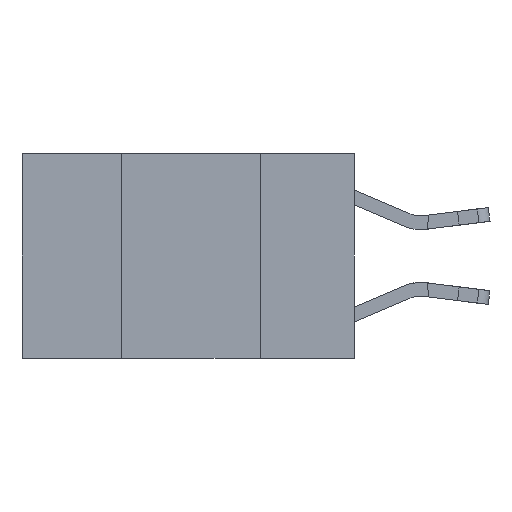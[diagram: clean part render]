
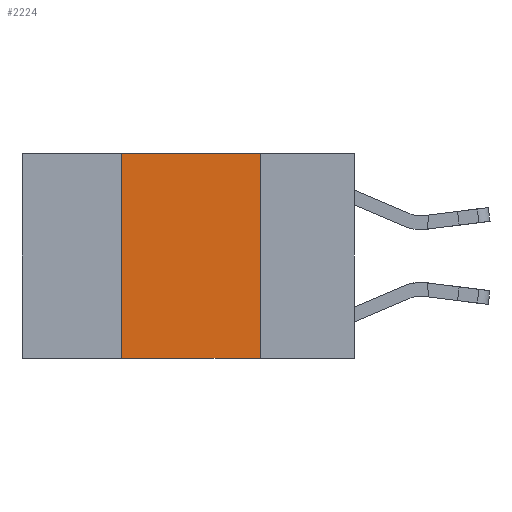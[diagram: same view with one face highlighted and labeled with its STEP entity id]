
A CAD part, left-side view. The second image highlights one B-rep face of the part: STEP entity #2224.
In plain terms, the highlighted planar face has unit normal (-1, 0, 0).
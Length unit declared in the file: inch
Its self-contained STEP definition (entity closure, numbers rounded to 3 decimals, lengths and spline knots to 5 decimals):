
#190 = CARTESIAN_POINT ( 'NONE',  ( 0., 0.17, -0.37 ) ) ;
#291 = VECTOR ( 'NONE', #15380, 39.37008 ) ;
#1201 = AXIS2_PLACEMENT_3D ( 'NONE', #17221, #19103, #23726 ) ;
#1230 = VERTEX_POINT ( 'NONE', #17264 ) ;
#2224 = ADVANCED_FACE ( 'NONE', ( #10831 ), #8373, .F. ) ;
#3230 = EDGE_CURVE ( 'NONE', #23734, #20694, #17258, .T. ) ;
#4207 = ORIENTED_EDGE ( 'NONE', *, *, #10523, .T. ) ;
#4534 = ORIENTED_EDGE ( 'NONE', *, *, #9745, .F. ) ;
#5258 = CARTESIAN_POINT ( 'NONE',  ( 0., 0.6, -0.37 ) ) ;
#7089 = EDGE_CURVE ( 'NONE', #1230, #23734, #14463, .T. ) ;
#7967 = DIRECTION ( 'NONE',  ( 0., 0., -1. ) ) ;
#8149 = VECTOR ( 'NONE', #11794, 39.37008 ) ;
#8373 = PLANE ( 'NONE',  #1201 ) ;
#9656 = VECTOR ( 'NONE', #12144, 39.37008 ) ;
#9745 = EDGE_CURVE ( 'NONE', #20694, #28521, #10006, .T. ) ;
#10006 = LINE ( 'NONE', #21170, #26594 ) ;
#10279 = ORIENTED_EDGE ( 'NONE', *, *, #7089, .F. ) ;
#10523 = EDGE_CURVE ( 'NONE', #1230, #28521, #13691, .T. ) ;
#10831 = FACE_OUTER_BOUND ( 'NONE', #28191, .T. ) ;
#11794 = DIRECTION ( 'NONE',  ( 0., -1., 0. ) ) ;
#12144 = DIRECTION ( 'NONE',  ( 0., 0., 1. ) ) ;
#13691 = LINE ( 'NONE', #5258, #8149 ) ;
#14463 = LINE ( 'NONE', #27887, #9656 ) ;
#14484 = ORIENTED_EDGE ( 'NONE', *, *, #3230, .F. ) ;
#15380 = DIRECTION ( 'NONE',  ( 0., -1., 0. ) ) ;
#16407 = CARTESIAN_POINT ( 'NONE',  ( 0., 0.42, 0. ) ) ;
#17221 = CARTESIAN_POINT ( 'NONE',  ( 0., 0.6, 0. ) ) ;
#17258 = LINE ( 'NONE', #19578, #291 ) ;
#17264 = CARTESIAN_POINT ( 'NONE',  ( 0., 0.42, -0.37 ) ) ;
#19103 = DIRECTION ( 'NONE',  ( 1., 0., 0. ) ) ;
#19578 = CARTESIAN_POINT ( 'NONE',  ( 0., 0.6, 0. ) ) ;
#20694 = VERTEX_POINT ( 'NONE', #27806 ) ;
#21170 = CARTESIAN_POINT ( 'NONE',  ( 0., 0.17, 0. ) ) ;
#23726 = DIRECTION ( 'NONE',  ( 0., 0., -1. ) ) ;
#23734 = VERTEX_POINT ( 'NONE', #16407 ) ;
#26594 = VECTOR ( 'NONE', #7967, 39.37008 ) ;
#27806 = CARTESIAN_POINT ( 'NONE',  ( 0., 0.17, 0. ) ) ;
#27887 = CARTESIAN_POINT ( 'NONE',  ( 0., 0.42, 0. ) ) ;
#28191 = EDGE_LOOP ( 'NONE', ( #4534, #14484, #10279, #4207 ) ) ;
#28521 = VERTEX_POINT ( 'NONE', #190 ) ;
